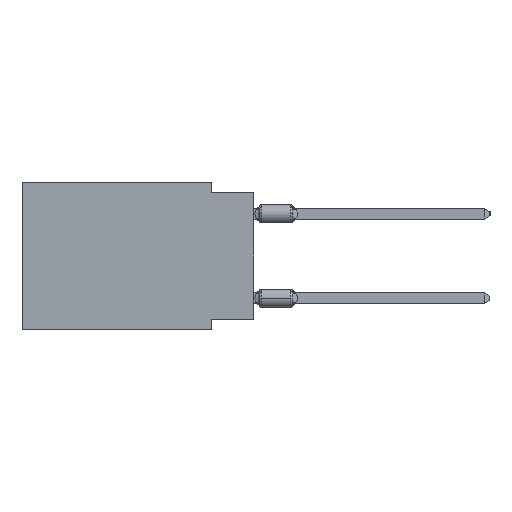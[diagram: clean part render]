
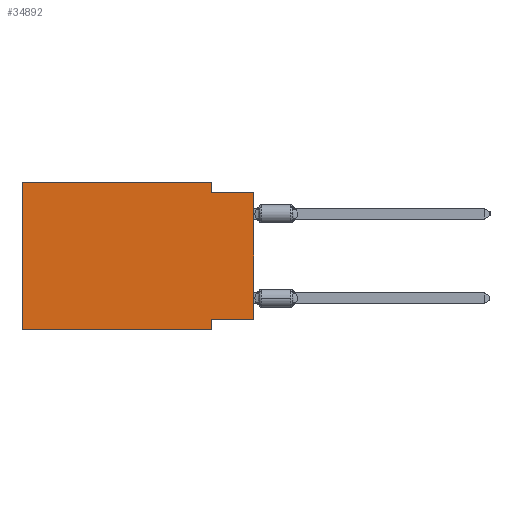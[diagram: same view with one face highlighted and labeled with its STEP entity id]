
A CAD part, left-side view. The second image highlights one B-rep face of the part: STEP entity #34892.
In plain terms, the highlighted planar face has unit normal (-1, 0, 0).
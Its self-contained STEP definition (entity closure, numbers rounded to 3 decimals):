
#1187 = LINE ( 'NONE', #34925, #47339 ) ;
#2410 = VECTOR ( 'NONE', #12108, 1000. ) ;
#2427 = CARTESIAN_POINT ( 'NONE',  ( 0., 0., -0.635 ) ) ;
#3068 = CARTESIAN_POINT ( 'NONE',  ( 0., 13.97, 0. ) ) ;
#3218 = ORIENTED_EDGE ( 'NONE', *, *, #19017, .F. ) ;
#3452 = CARTESIAN_POINT ( 'NONE',  ( 0., 13.97, -8.89 ) ) ;
#3853 = VECTOR ( 'NONE', #44833, 1000. ) ;
#4127 = ORIENTED_EDGE ( 'NONE', *, *, #30402, .F. ) ;
#6006 = VERTEX_POINT ( 'NONE', #39001 ) ;
#6908 = VECTOR ( 'NONE', #24500, 1000. ) ;
#6961 = VERTEX_POINT ( 'NONE', #38137 ) ;
#7884 = DIRECTION ( 'NONE',  ( 0., -1., 0. ) ) ;
#8775 = VERTEX_POINT ( 'NONE', #3452 ) ;
#9068 = VECTOR ( 'NONE', #7884, 1000. ) ;
#10387 = CARTESIAN_POINT ( 'NONE',  ( 0., 2.54, -0.635 ) ) ;
#11483 = AXIS2_PLACEMENT_3D ( 'NONE', #16672, #12993, #27891 ) ;
#12108 = DIRECTION ( 'NONE',  ( 0., 1., 0. ) ) ;
#12135 = CARTESIAN_POINT ( 'NONE',  ( 0., 2.54, 0. ) ) ;
#12551 = CARTESIAN_POINT ( 'NONE',  ( 0., 0., 0. ) ) ;
#12993 = DIRECTION ( 'NONE',  ( 1., 0., 0. ) ) ;
#14286 = LINE ( 'NONE', #33335, #26177 ) ;
#15866 = ORIENTED_EDGE ( 'NONE', *, *, #40863, .F. ) ;
#16219 = VECTOR ( 'NONE', #23263, 1000. ) ;
#16672 = CARTESIAN_POINT ( 'NONE',  ( 0., 13.97, 0. ) ) ;
#16675 = VERTEX_POINT ( 'NONE', #10387 ) ;
#19017 = EDGE_CURVE ( 'NONE', #37329, #6961, #23095, .T. ) ;
#19175 = CARTESIAN_POINT ( 'NONE',  ( 0., 2.54, 0. ) ) ;
#22274 = EDGE_CURVE ( 'NONE', #37329, #44690, #31102, .T. ) ;
#22975 = ORIENTED_EDGE ( 'NONE', *, *, #40331, .F. ) ;
#23092 = CARTESIAN_POINT ( 'NONE',  ( 0., 13.97, 0. ) ) ;
#23095 = LINE ( 'NONE', #37541, #2410 ) ;
#23263 = DIRECTION ( 'NONE',  ( 0., 0., -1. ) ) ;
#24199 = VECTOR ( 'NONE', #31939, 1000. ) ;
#24500 = DIRECTION ( 'NONE',  ( 0., 0., 1. ) ) ;
#24837 = VERTEX_POINT ( 'NONE', #23092 ) ;
#26177 = VECTOR ( 'NONE', #48242, 1000. ) ;
#27891 = DIRECTION ( 'NONE',  ( 0., 0., -1. ) ) ;
#29649 = ORIENTED_EDGE ( 'NONE', *, *, #22274, .T. ) ;
#30402 = EDGE_CURVE ( 'NONE', #6961, #6006, #42570, .T. ) ;
#31102 = LINE ( 'NONE', #12551, #6908 ) ;
#31939 = DIRECTION ( 'NONE',  ( 0., -1., 0. ) ) ;
#33024 = EDGE_CURVE ( 'NONE', #48098, #16675, #37267, .T. ) ;
#33335 = CARTESIAN_POINT ( 'NONE',  ( 0., 13.97, -8.89 ) ) ;
#33648 = EDGE_LOOP ( 'NONE', ( #29649, #22975, #44129, #38803, #15866, #38578, #4127, #3218 ) ) ;
#34029 = CARTESIAN_POINT ( 'NONE',  ( 0., 0., -0.635 ) ) ;
#34892 = ADVANCED_FACE ( 'NONE', ( #40096 ), #35707, .F. ) ;
#34925 = CARTESIAN_POINT ( 'NONE',  ( 0., 13.97, 0. ) ) ;
#35707 = PLANE ( 'NONE',  #11483 ) ;
#36561 = LINE ( 'NONE', #3068, #24199 ) ;
#37267 = LINE ( 'NONE', #19175, #3853 ) ;
#37329 = VERTEX_POINT ( 'NONE', #40955 ) ;
#37541 = CARTESIAN_POINT ( 'NONE',  ( 0., 0., -8.255 ) ) ;
#38137 = CARTESIAN_POINT ( 'NONE',  ( 0., 2.54, -8.255 ) ) ;
#38578 = ORIENTED_EDGE ( 'NONE', *, *, #39180, .T. ) ;
#38803 = ORIENTED_EDGE ( 'NONE', *, *, #42705, .F. ) ;
#38889 = CARTESIAN_POINT ( 'NONE',  ( 0., 2.54, -8.89 ) ) ;
#39001 = CARTESIAN_POINT ( 'NONE',  ( 0., 2.54, -8.89 ) ) ;
#39180 = EDGE_CURVE ( 'NONE', #8775, #6006, #14286, .T. ) ;
#40096 = FACE_OUTER_BOUND ( 'NONE', #33648, .T. ) ;
#40331 = EDGE_CURVE ( 'NONE', #16675, #44690, #45028, .T. ) ;
#40863 = EDGE_CURVE ( 'NONE', #8775, #24837, #1187, .T. ) ;
#40955 = CARTESIAN_POINT ( 'NONE',  ( 0., 0., -8.255 ) ) ;
#42570 = LINE ( 'NONE', #38889, #16219 ) ;
#42705 = EDGE_CURVE ( 'NONE', #24837, #48098, #36561, .T. ) ;
#44129 = ORIENTED_EDGE ( 'NONE', *, *, #33024, .F. ) ;
#44690 = VERTEX_POINT ( 'NONE', #2427 ) ;
#44833 = DIRECTION ( 'NONE',  ( 0., 0., -1. ) ) ;
#45028 = LINE ( 'NONE', #34029, #9068 ) ;
#45930 = DIRECTION ( 'NONE',  ( 0., 0., 1. ) ) ;
#47339 = VECTOR ( 'NONE', #45930, 1000. ) ;
#48098 = VERTEX_POINT ( 'NONE', #12135 ) ;
#48242 = DIRECTION ( 'NONE',  ( 0., -1., 0. ) ) ;
